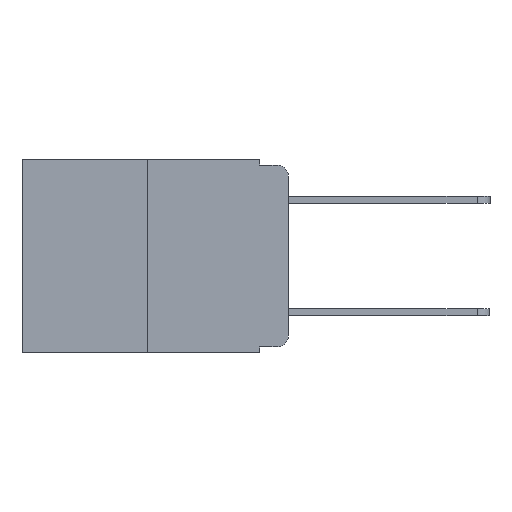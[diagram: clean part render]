
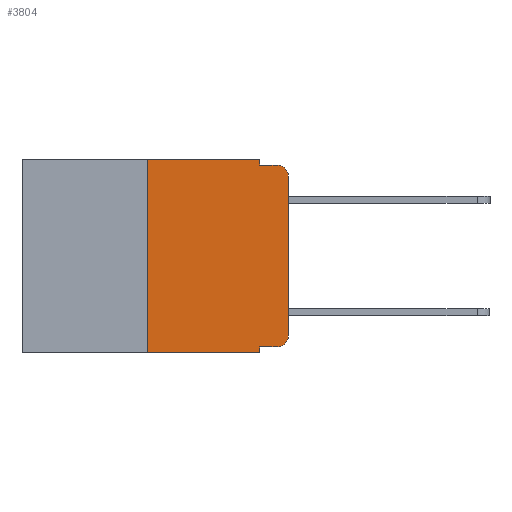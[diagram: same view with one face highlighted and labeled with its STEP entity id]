
A CAD part, left-side view. The second image highlights one B-rep face of the part: STEP entity #3804.
In plain terms, the highlighted planar face has unit normal (-1, 0, 0).
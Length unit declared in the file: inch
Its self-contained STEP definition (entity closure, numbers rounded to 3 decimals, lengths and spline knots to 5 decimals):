
#209 = DIRECTION ( 'NONE',  ( 0., 0., 1. ) ) ;
#247 = AXIS2_PLACEMENT_3D ( 'NONE', #6754, #11152, #2293 ) ;
#325 = DIRECTION ( 'NONE',  ( -1., 0., 0. ) ) ;
#654 = CARTESIAN_POINT ( 'NONE',  ( 0., 0.051, -0.01 ) ) ;
#839 = CIRCLE ( 'NONE', #3000, 0.02 ) ;
#1270 = CARTESIAN_POINT ( 'NONE',  ( 0., 0., -0.03 ) ) ;
#1563 = VERTEX_POINT ( 'NONE', #12153 ) ;
#1765 = VERTEX_POINT ( 'NONE', #4100 ) ;
#1828 = ORIENTED_EDGE ( 'NONE', *, *, #12178, .T. ) ;
#2293 = DIRECTION ( 'NONE',  ( 0., 0., -1. ) ) ;
#2383 = DIRECTION ( 'NONE',  ( 0., -1., 0. ) ) ;
#2585 = EDGE_CURVE ( 'NONE', #14267, #3278, #18001, .T. ) ;
#2610 = CARTESIAN_POINT ( 'NONE',  ( 0., 0.051, -0.333 ) ) ;
#2782 = LINE ( 'NONE', #15519, #6306 ) ;
#3000 = AXIS2_PLACEMENT_3D ( 'NONE', #6907, #16757, #8407 ) ;
#3004 = ORIENTED_EDGE ( 'NONE', *, *, #5257, .F. ) ;
#3092 = CARTESIAN_POINT ( 'NONE',  ( 0., 0.02, -0.333 ) ) ;
#3161 = EDGE_LOOP ( 'NONE', ( #4637, #16851, #3004, #6280, #10640, #8590, #12789, #6511, #7894, #1828 ) ) ;
#3278 = VERTEX_POINT ( 'NONE', #6833 ) ;
#3418 = VECTOR ( 'NONE', #13208, 39.37008 ) ;
#3804 = ADVANCED_FACE ( 'NONE', ( #7113 ), #9733, .F. ) ;
#3901 = VECTOR ( 'NONE', #2383, 39.37008 ) ;
#4100 = CARTESIAN_POINT ( 'NONE',  ( 0., 0.051, 0. ) ) ;
#4141 = CARTESIAN_POINT ( 'NONE',  ( 0., 0.473, -0.343 ) ) ;
#4554 = EDGE_CURVE ( 'NONE', #7948, #1765, #16370, .T. ) ;
#4556 = VERTEX_POINT ( 'NONE', #8073 ) ;
#4637 = ORIENTED_EDGE ( 'NONE', *, *, #9476, .T. ) ;
#5100 = CARTESIAN_POINT ( 'NONE',  ( 0., 0.473, 0. ) ) ;
#5257 = EDGE_CURVE ( 'NONE', #1563, #9968, #8687, .T. ) ;
#5621 = DIRECTION ( 'NONE',  ( 0., -1., 0. ) ) ;
#5853 = VECTOR ( 'NONE', #209, 39.37008 ) ;
#5956 = VECTOR ( 'NONE', #15023, 39.37008 ) ;
#5977 = VECTOR ( 'NONE', #5621, 39.37008 ) ;
#6280 = ORIENTED_EDGE ( 'NONE', *, *, #14244, .F. ) ;
#6306 = VECTOR ( 'NONE', #8553, 39.37008 ) ;
#6424 = DIRECTION ( 'NONE',  ( 0., 0., -1. ) ) ;
#6511 = ORIENTED_EDGE ( 'NONE', *, *, #2585, .F. ) ;
#6602 = EDGE_CURVE ( 'NONE', #13055, #7948, #7340, .T. ) ;
#6754 = CARTESIAN_POINT ( 'NONE',  ( 0., 0.473, 0. ) ) ;
#6833 = CARTESIAN_POINT ( 'NONE',  ( 0., 0.051, -0.343 ) ) ;
#6907 = CARTESIAN_POINT ( 'NONE',  ( 0., 0.02, -0.313 ) ) ;
#7113 = FACE_OUTER_BOUND ( 'NONE', #3161, .T. ) ;
#7340 = LINE ( 'NONE', #11830, #3418 ) ;
#7894 = ORIENTED_EDGE ( 'NONE', *, *, #16751, .T. ) ;
#7948 = VERTEX_POINT ( 'NONE', #14706 ) ;
#8073 = CARTESIAN_POINT ( 'NONE',  ( 0., 0., -0.313 ) ) ;
#8211 = EDGE_CURVE ( 'NONE', #18117, #9968, #15468, .T. ) ;
#8215 = VECTOR ( 'NONE', #17871, 39.37008 ) ;
#8407 = DIRECTION ( 'NONE',  ( 0., 0., -1. ) ) ;
#8553 = DIRECTION ( 'NONE',  ( 0., 0., -1. ) ) ;
#8590 = ORIENTED_EDGE ( 'NONE', *, *, #6602, .F. ) ;
#8687 = LINE ( 'NONE', #654, #8215 ) ;
#9161 = CARTESIAN_POINT ( 'NONE',  ( 0., 0., 0. ) ) ;
#9264 = CARTESIAN_POINT ( 'NONE',  ( 0., 0.02, -0.03 ) ) ;
#9476 = EDGE_CURVE ( 'NONE', #4556, #18117, #9770, .T. ) ;
#9733 = PLANE ( 'NONE',  #247 ) ;
#9770 = LINE ( 'NONE', #9161, #5853 ) ;
#9968 = VERTEX_POINT ( 'NONE', #17069 ) ;
#10640 = ORIENTED_EDGE ( 'NONE', *, *, #4554, .F. ) ;
#10714 = DIRECTION ( 'NONE',  ( 0., 0., -1. ) ) ;
#11152 = DIRECTION ( 'NONE',  ( 1., 0., 0. ) ) ;
#11830 = CARTESIAN_POINT ( 'NONE',  ( 0., 0.25, 0. ) ) ;
#12153 = CARTESIAN_POINT ( 'NONE',  ( 0., 0.051, -0.01 ) ) ;
#12178 = EDGE_CURVE ( 'NONE', #14501, #4556, #839, .T. ) ;
#12521 = LINE ( 'NONE', #14014, #3901 ) ;
#12789 = ORIENTED_EDGE ( 'NONE', *, *, #16849, .T. ) ;
#13055 = VERTEX_POINT ( 'NONE', #18218 ) ;
#13208 = DIRECTION ( 'NONE',  ( 0., 0., 1. ) ) ;
#13597 = LINE ( 'NONE', #4141, #5977 ) ;
#14014 = CARTESIAN_POINT ( 'NONE',  ( 0., 0.051, -0.333 ) ) ;
#14244 = EDGE_CURVE ( 'NONE', #1765, #1563, #2782, .T. ) ;
#14267 = VERTEX_POINT ( 'NONE', #2610 ) ;
#14501 = VERTEX_POINT ( 'NONE', #3092 ) ;
#14706 = CARTESIAN_POINT ( 'NONE',  ( 0., 0.25, 0. ) ) ;
#14790 = VECTOR ( 'NONE', #6424, 39.37008 ) ;
#14933 = CARTESIAN_POINT ( 'NONE',  ( 0., 0.051, 0. ) ) ;
#15023 = DIRECTION ( 'NONE',  ( 0., -1., 0. ) ) ;
#15468 = CIRCLE ( 'NONE', #18220, 0.02 ) ;
#15519 = CARTESIAN_POINT ( 'NONE',  ( 0., 0.051, 0. ) ) ;
#16370 = LINE ( 'NONE', #5100, #5956 ) ;
#16751 = EDGE_CURVE ( 'NONE', #14267, #14501, #12521, .T. ) ;
#16757 = DIRECTION ( 'NONE',  ( -1., 0., 0. ) ) ;
#16849 = EDGE_CURVE ( 'NONE', #13055, #3278, #13597, .T. ) ;
#16851 = ORIENTED_EDGE ( 'NONE', *, *, #8211, .T. ) ;
#17069 = CARTESIAN_POINT ( 'NONE',  ( 0., 0.02, -0.01 ) ) ;
#17871 = DIRECTION ( 'NONE',  ( 0., -1., 0. ) ) ;
#18001 = LINE ( 'NONE', #14933, #14790 ) ;
#18117 = VERTEX_POINT ( 'NONE', #1270 ) ;
#18218 = CARTESIAN_POINT ( 'NONE',  ( 0., 0.25, -0.343 ) ) ;
#18220 = AXIS2_PLACEMENT_3D ( 'NONE', #9264, #325, #10714 ) ;
